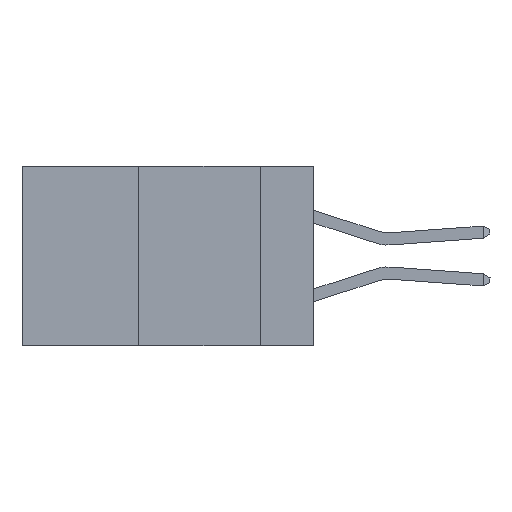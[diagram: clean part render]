
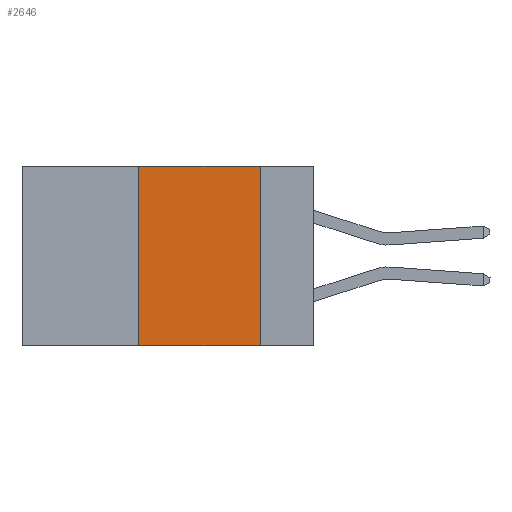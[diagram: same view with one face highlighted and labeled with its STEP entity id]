
A CAD part, left-side view. The second image highlights one B-rep face of the part: STEP entity #2646.
In plain terms, the highlighted planar face has unit normal (-1, 0, 0).
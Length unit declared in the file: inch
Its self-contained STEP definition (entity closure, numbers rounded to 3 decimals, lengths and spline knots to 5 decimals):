
#512 = CARTESIAN_POINT ( 'NONE',  ( 0., 0.6, 0. ) ) ;
#1725 = CARTESIAN_POINT ( 'NONE',  ( 0., 0.11, 0. ) ) ;
#2120 = ORIENTED_EDGE ( 'NONE', *, *, #12173, .T. ) ;
#2646 = ADVANCED_FACE ( 'NONE', ( #5771 ), #9449, .F. ) ;
#2808 = VECTOR ( 'NONE', #3564, 39.37008 ) ;
#2989 = VERTEX_POINT ( 'NONE', #5686 ) ;
#3564 = DIRECTION ( 'NONE',  ( 0., 0., 1. ) ) ;
#4277 = LINE ( 'NONE', #1725, #8814 ) ;
#4672 = ORIENTED_EDGE ( 'NONE', *, *, #16303, .F. ) ;
#5686 = CARTESIAN_POINT ( 'NONE',  ( 0., 0.11, 0. ) ) ;
#5771 = FACE_OUTER_BOUND ( 'NONE', #14875, .T. ) ;
#6139 = CARTESIAN_POINT ( 'NONE',  ( 0., 0.36, 0. ) ) ;
#6531 = CARTESIAN_POINT ( 'NONE',  ( 0., 0.6, -0.37 ) ) ;
#7907 = DIRECTION ( 'NONE',  ( 0., 0., -1. ) ) ;
#8797 = CARTESIAN_POINT ( 'NONE',  ( 0., 0.11, -0.37 ) ) ;
#8814 = VECTOR ( 'NONE', #11956, 39.37008 ) ;
#9449 = PLANE ( 'NONE',  #11856 ) ;
#9646 = DIRECTION ( 'NONE',  ( 1., 0., 0. ) ) ;
#9690 = VECTOR ( 'NONE', #20845, 39.37008 ) ;
#10539 = EDGE_CURVE ( 'NONE', #20529, #2989, #14747, .T. ) ;
#10701 = LINE ( 'NONE', #6531, #20167 ) ;
#11751 = VERTEX_POINT ( 'NONE', #8797 ) ;
#11856 = AXIS2_PLACEMENT_3D ( 'NONE', #14695, #9646, #7907 ) ;
#11956 = DIRECTION ( 'NONE',  ( 0., 0., -1. ) ) ;
#12173 = EDGE_CURVE ( 'NONE', #13264, #11751, #10701, .T. ) ;
#12386 = ORIENTED_EDGE ( 'NONE', *, *, #18701, .F. ) ;
#13264 = VERTEX_POINT ( 'NONE', #19752 ) ;
#14695 = CARTESIAN_POINT ( 'NONE',  ( 0., 0.6, 0. ) ) ;
#14747 = LINE ( 'NONE', #512, #9690 ) ;
#14875 = EDGE_LOOP ( 'NONE', ( #4672, #18105, #12386, #2120 ) ) ;
#15019 = DIRECTION ( 'NONE',  ( 0., -1., 0. ) ) ;
#16303 = EDGE_CURVE ( 'NONE', #2989, #11751, #4277, .T. ) ;
#18105 = ORIENTED_EDGE ( 'NONE', *, *, #10539, .F. ) ;
#18701 = EDGE_CURVE ( 'NONE', #13264, #20529, #20870, .T. ) ;
#18762 = CARTESIAN_POINT ( 'NONE',  ( 0., 0.36, 0. ) ) ;
#19752 = CARTESIAN_POINT ( 'NONE',  ( 0., 0.36, -0.37 ) ) ;
#20167 = VECTOR ( 'NONE', #15019, 39.37008 ) ;
#20529 = VERTEX_POINT ( 'NONE', #6139 ) ;
#20845 = DIRECTION ( 'NONE',  ( 0., -1., 0. ) ) ;
#20870 = LINE ( 'NONE', #18762, #2808 ) ;
